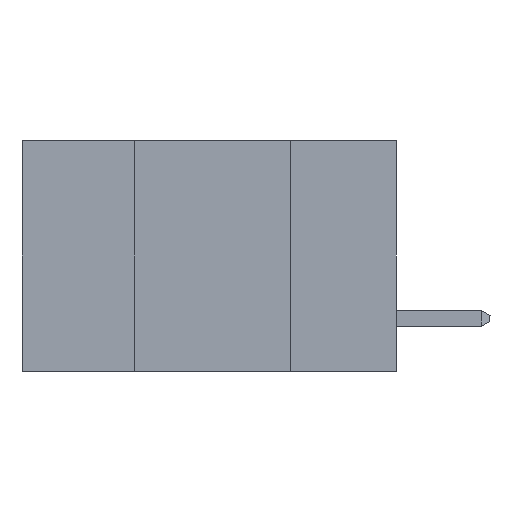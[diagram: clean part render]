
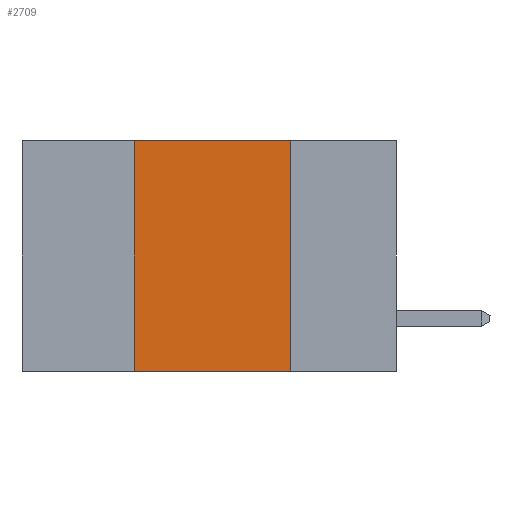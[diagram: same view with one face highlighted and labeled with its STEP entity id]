
A CAD part, left-side view. The second image highlights one B-rep face of the part: STEP entity #2709.
In plain terms, the highlighted planar face has unit normal (-1, 0, 0).
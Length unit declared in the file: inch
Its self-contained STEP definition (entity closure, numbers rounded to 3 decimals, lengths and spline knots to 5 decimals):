
#938 = DIRECTION ( 'NONE',  ( 0., -1., 0. ) ) ;
#958 = VECTOR ( 'NONE', #3165, 39.37008 ) ;
#2102 = EDGE_LOOP ( 'NONE', ( #12714, #7796, #2168, #11091 ) ) ;
#2168 = ORIENTED_EDGE ( 'NONE', *, *, #4438, .F. ) ;
#2644 = DIRECTION ( 'NONE',  ( 0., 0., -1. ) ) ;
#2709 = ADVANCED_FACE ( 'NONE', ( #3777 ), #9229, .F. ) ;
#2864 = VERTEX_POINT ( 'NONE', #13999 ) ;
#3090 = EDGE_CURVE ( 'NONE', #12569, #2864, #6524, .T. ) ;
#3165 = DIRECTION ( 'NONE',  ( 0., 0., 1. ) ) ;
#3418 = LINE ( 'NONE', #16949, #5626 ) ;
#3594 = CARTESIAN_POINT ( 'NONE',  ( 0., 0.6, 0. ) ) ;
#3777 = FACE_OUTER_BOUND ( 'NONE', #2102, .T. ) ;
#4438 = EDGE_CURVE ( 'NONE', #9970, #11305, #7235, .T. ) ;
#4853 = LINE ( 'NONE', #8750, #8645 ) ;
#5626 = VECTOR ( 'NONE', #938, 39.37008 ) ;
#6524 = LINE ( 'NONE', #16112, #7911 ) ;
#6666 = CARTESIAN_POINT ( 'NONE',  ( 0., 0.17, 0. ) ) ;
#7235 = LINE ( 'NONE', #12751, #958 ) ;
#7365 = EDGE_CURVE ( 'NONE', #11305, #12569, #4853, .T. ) ;
#7796 = ORIENTED_EDGE ( 'NONE', *, *, #7365, .F. ) ;
#7839 = AXIS2_PLACEMENT_3D ( 'NONE', #3594, #9313, #7904 ) ;
#7904 = DIRECTION ( 'NONE',  ( 0., 0., -1. ) ) ;
#7911 = VECTOR ( 'NONE', #2644, 39.37008 ) ;
#8645 = VECTOR ( 'NONE', #11641, 39.37008 ) ;
#8750 = CARTESIAN_POINT ( 'NONE',  ( 0., 0.6, 0. ) ) ;
#9229 = PLANE ( 'NONE',  #7839 ) ;
#9313 = DIRECTION ( 'NONE',  ( 1., 0., 0. ) ) ;
#9970 = VERTEX_POINT ( 'NONE', #13758 ) ;
#11091 = ORIENTED_EDGE ( 'NONE', *, *, #12425, .T. ) ;
#11305 = VERTEX_POINT ( 'NONE', #12643 ) ;
#11641 = DIRECTION ( 'NONE',  ( 0., -1., 0. ) ) ;
#12425 = EDGE_CURVE ( 'NONE', #9970, #2864, #3418, .T. ) ;
#12569 = VERTEX_POINT ( 'NONE', #6666 ) ;
#12643 = CARTESIAN_POINT ( 'NONE',  ( 0., 0.42, 0. ) ) ;
#12714 = ORIENTED_EDGE ( 'NONE', *, *, #3090, .F. ) ;
#12751 = CARTESIAN_POINT ( 'NONE',  ( 0., 0.42, -0.37 ) ) ;
#13758 = CARTESIAN_POINT ( 'NONE',  ( 0., 0.42, -0.37 ) ) ;
#13999 = CARTESIAN_POINT ( 'NONE',  ( 0., 0.17, -0.37 ) ) ;
#16112 = CARTESIAN_POINT ( 'NONE',  ( 0., 0.17, -0.37 ) ) ;
#16949 = CARTESIAN_POINT ( 'NONE',  ( 0., 0.6, -0.37 ) ) ;
